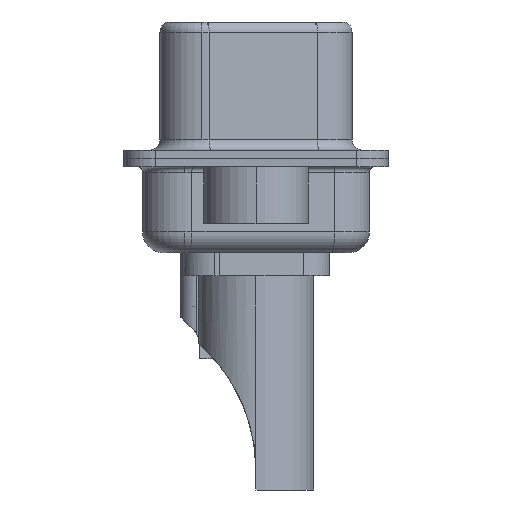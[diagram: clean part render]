
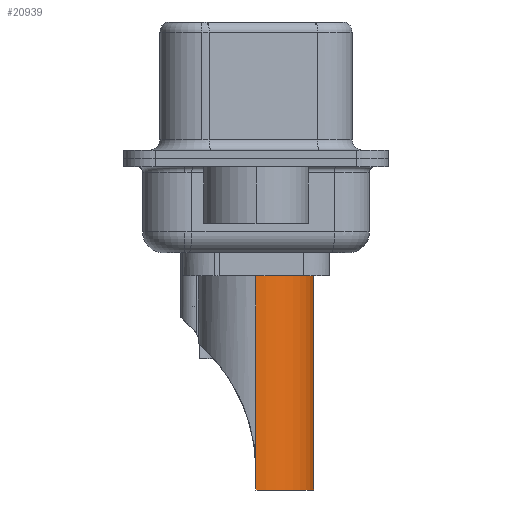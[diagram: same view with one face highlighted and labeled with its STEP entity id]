
A CAD part, left-side view. The second image highlights one B-rep face of the part: STEP entity #20939.
In plain terms, the highlighted cylindrical face has radius 2.75 mm (diameter 5.5 mm), a partial arc.
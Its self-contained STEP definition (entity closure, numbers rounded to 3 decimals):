
#457 = LINE ( 'NONE', #18110, #13558 ) ;
#681 = EDGE_CURVE ( 'NONE', #19986, #5290, #4744, .T. ) ;
#1771 = CARTESIAN_POINT ( 'NONE',  ( -2.75, 0., -7.764 ) ) ;
#2383 = VERTEX_POINT ( 'NONE', #7252 ) ;
#2496 = ORIENTED_EDGE ( 'NONE', *, *, #681, .F. ) ;
#2528 = DIRECTION ( 'NONE',  ( 0., 0., -1. ) ) ;
#2945 = CARTESIAN_POINT ( 'NONE',  ( 2.75, 0., -8.7 ) ) ;
#3087 = CARTESIAN_POINT ( 'NONE',  ( 2.75, 0., -7.764 ) ) ;
#3999 = CARTESIAN_POINT ( 'NONE',  ( 2.75, 0., -8.7 ) ) ;
#4744 = LINE ( 'NONE', #2945, #8959 ) ;
#4843 = VECTOR ( 'NONE', #18841, 1000. ) ;
#4947 = AXIS2_PLACEMENT_3D ( 'NONE', #10845, #19597, #16125 ) ;
#5177 = ORIENTED_EDGE ( 'NONE', *, *, #9908, .T. ) ;
#5240 = DIRECTION ( 'NONE',  ( 0., 0., 1. ) ) ;
#5290 = VERTEX_POINT ( 'NONE', #3999 ) ;
#5659 = DIRECTION ( 'NONE',  ( 0., 0., 1. ) ) ;
#6805 = CARTESIAN_POINT ( 'NONE',  ( 0., 0., -8.7 ) ) ;
#7252 = CARTESIAN_POINT ( 'NONE',  ( 2.75, 0., 1.5 ) ) ;
#7624 = VECTOR ( 'NONE', #5659, 1000. ) ;
#7641 = VERTEX_POINT ( 'NONE', #16549 ) ;
#8631 = DIRECTION ( 'NONE',  ( 1., 0., 0. ) ) ;
#8739 = AXIS2_PLACEMENT_3D ( 'NONE', #15807, #5240, #17533 ) ;
#8741 = ORIENTED_EDGE ( 'NONE', *, *, #10325, .T. ) ;
#8959 = VECTOR ( 'NONE', #2528, 1000. ) ;
#9247 = CARTESIAN_POINT ( 'NONE',  ( 2.75, 0., 4.234 ) ) ;
#9310 = CARTESIAN_POINT ( 'NONE',  ( -2.75, 0., -8.7 ) ) ;
#9693 = ORIENTED_EDGE ( 'NONE', *, *, #18540, .T. ) ;
#9908 = EDGE_CURVE ( 'NONE', #19986, #2383, #22000, .T. ) ;
#10325 = EDGE_CURVE ( 'NONE', #18056, #5290, #13254, .T. ) ;
#10845 = CARTESIAN_POINT ( 'NONE',  ( 0., 0., 4.234 ) ) ;
#11854 = AXIS2_PLACEMENT_3D ( 'NONE', #6805, #19029, #8631 ) ;
#12459 = EDGE_LOOP ( 'NONE', ( #22697, #9693, #8741, #2496, #5177, #17780 ) ) ;
#12631 = CYLINDRICAL_SURFACE ( 'NONE', #4947, 2.75 ) ;
#13254 = CIRCLE ( 'NONE', #11854, 2.75 ) ;
#13558 = VECTOR ( 'NONE', #16379, 1000. ) ;
#15362 = CARTESIAN_POINT ( 'NONE',  ( -2.75, 0., 4.234 ) ) ;
#15784 = EDGE_CURVE ( 'NONE', #20199, #7641, #18859, .T. ) ;
#15807 = CARTESIAN_POINT ( 'NONE',  ( 0., 0., 1.5 ) ) ;
#16125 = DIRECTION ( 'NONE',  ( 1., 0., 0. ) ) ;
#16379 = DIRECTION ( 'NONE',  ( 0., 0., -1. ) ) ;
#16549 = CARTESIAN_POINT ( 'NONE',  ( -2.75, 0., 1.5 ) ) ;
#17533 = DIRECTION ( 'NONE',  ( 1., 0., 0. ) ) ;
#17780 = ORIENTED_EDGE ( 'NONE', *, *, #22417, .F. ) ;
#18056 = VERTEX_POINT ( 'NONE', #9310 ) ;
#18075 = CIRCLE ( 'NONE', #8739, 2.75 ) ;
#18110 = CARTESIAN_POINT ( 'NONE',  ( -2.75, 0., -8.7 ) ) ;
#18540 = EDGE_CURVE ( 'NONE', #20199, #18056, #457, .T. ) ;
#18841 = DIRECTION ( 'NONE',  ( 0., 0., 1. ) ) ;
#18859 = LINE ( 'NONE', #15362, #4843 ) ;
#19029 = DIRECTION ( 'NONE',  ( 0., 0., 1. ) ) ;
#19597 = DIRECTION ( 'NONE',  ( 0., 0., 1. ) ) ;
#19986 = VERTEX_POINT ( 'NONE', #3087 ) ;
#20199 = VERTEX_POINT ( 'NONE', #1771 ) ;
#20939 = ADVANCED_FACE ( 'NONE', ( #22452 ), #12631, .T. ) ;
#22000 = LINE ( 'NONE', #9247, #7624 ) ;
#22417 = EDGE_CURVE ( 'NONE', #7641, #2383, #18075, .T. ) ;
#22452 = FACE_OUTER_BOUND ( 'NONE', #12459, .T. ) ;
#22697 = ORIENTED_EDGE ( 'NONE', *, *, #15784, .F. ) ;
